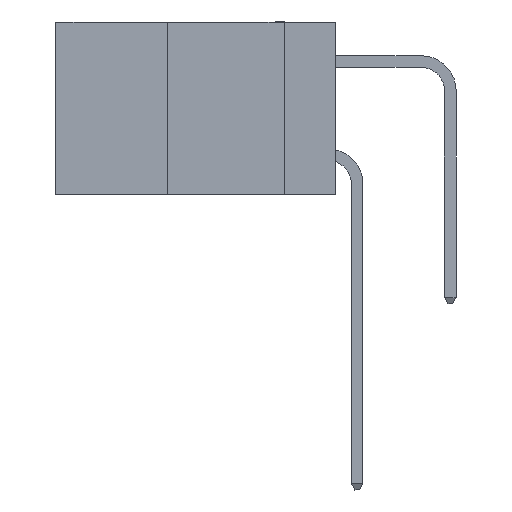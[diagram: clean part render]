
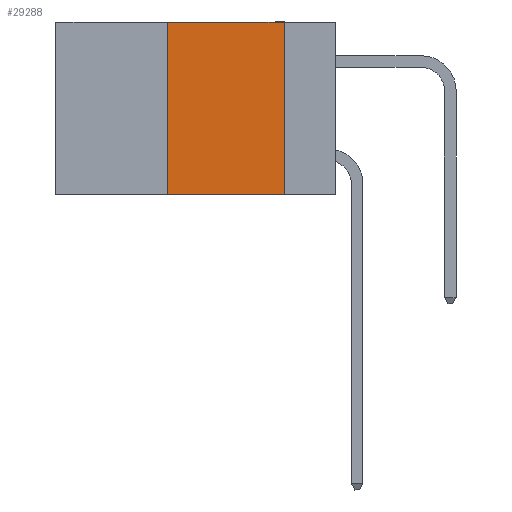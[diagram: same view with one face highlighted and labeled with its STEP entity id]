
A CAD part, left-side view. The second image highlights one B-rep face of the part: STEP entity #29288.
In plain terms, the highlighted planar face has unit normal (-1, 0, 0).
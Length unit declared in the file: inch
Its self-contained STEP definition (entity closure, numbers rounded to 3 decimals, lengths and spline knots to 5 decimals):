
#218 = LINE ( 'NONE', #17786, #27151 ) ;
#1557 = CARTESIAN_POINT ( 'NONE',  ( 0., 0.6, 0. ) ) ;
#2541 = AXIS2_PLACEMENT_3D ( 'NONE', #1557, #20659, #33584 ) ;
#4739 = CARTESIAN_POINT ( 'NONE',  ( 0., 0.6, -0.37 ) ) ;
#5109 = CARTESIAN_POINT ( 'NONE',  ( 0., 0.11, 0. ) ) ;
#6751 = FACE_OUTER_BOUND ( 'NONE', #13794, .T. ) ;
#10949 = LINE ( 'NONE', #13756, #27436 ) ;
#11397 = EDGE_CURVE ( 'NONE', #28845, #35521, #218, .T. ) ;
#12724 = VECTOR ( 'NONE', #17803, 39.37008 ) ;
#12800 = ORIENTED_EDGE ( 'NONE', *, *, #11397, .F. ) ;
#13756 = CARTESIAN_POINT ( 'NONE',  ( 0., 0.36, 0. ) ) ;
#13794 = EDGE_LOOP ( 'NONE', ( #37105, #12800, #15796, #23638 ) ) ;
#14365 = PLANE ( 'NONE',  #2541 ) ;
#14419 = CARTESIAN_POINT ( 'NONE',  ( 0., 0.11, -0.37 ) ) ;
#15796 = ORIENTED_EDGE ( 'NONE', *, *, #32601, .F. ) ;
#16292 = DIRECTION ( 'NONE',  ( 0., 0., 1. ) ) ;
#17786 = CARTESIAN_POINT ( 'NONE',  ( 0., 0.6, 0. ) ) ;
#17803 = DIRECTION ( 'NONE',  ( 0., 0., -1. ) ) ;
#18128 = DIRECTION ( 'NONE',  ( 0., -1., 0. ) ) ;
#19713 = VERTEX_POINT ( 'NONE', #14419 ) ;
#20465 = EDGE_CURVE ( 'NONE', #32035, #19713, #23051, .T. ) ;
#20659 = DIRECTION ( 'NONE',  ( 1., 0., 0. ) ) ;
#22196 = CARTESIAN_POINT ( 'NONE',  ( 0., 0.36, 0. ) ) ;
#23051 = LINE ( 'NONE', #4739, #26047 ) ;
#23251 = LINE ( 'NONE', #5109, #12724 ) ;
#23638 = ORIENTED_EDGE ( 'NONE', *, *, #20465, .T. ) ;
#24516 = CARTESIAN_POINT ( 'NONE',  ( 0., 0.11, 0. ) ) ;
#26047 = VECTOR ( 'NONE', #18128, 39.37008 ) ;
#27151 = VECTOR ( 'NONE', #31033, 39.37008 ) ;
#27436 = VECTOR ( 'NONE', #16292, 39.37008 ) ;
#28845 = VERTEX_POINT ( 'NONE', #22196 ) ;
#29288 = ADVANCED_FACE ( 'NONE', ( #6751 ), #14365, .F. ) ;
#29715 = CARTESIAN_POINT ( 'NONE',  ( 0., 0.36, -0.37 ) ) ;
#31033 = DIRECTION ( 'NONE',  ( 0., -1., 0. ) ) ;
#32035 = VERTEX_POINT ( 'NONE', #29715 ) ;
#32601 = EDGE_CURVE ( 'NONE', #32035, #28845, #10949, .T. ) ;
#33584 = DIRECTION ( 'NONE',  ( 0., 0., -1. ) ) ;
#35521 = VERTEX_POINT ( 'NONE', #24516 ) ;
#35549 = EDGE_CURVE ( 'NONE', #35521, #19713, #23251, .T. ) ;
#37105 = ORIENTED_EDGE ( 'NONE', *, *, #35549, .F. ) ;
